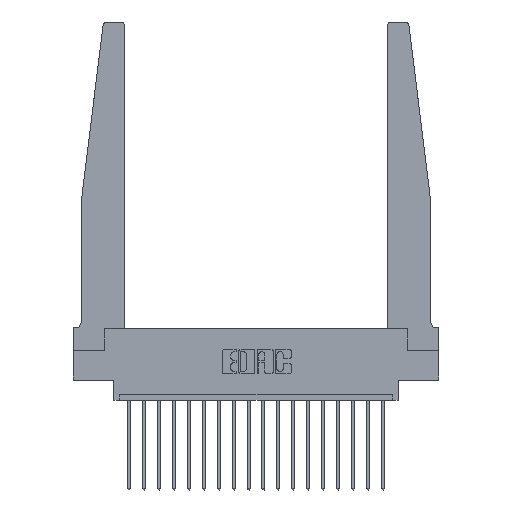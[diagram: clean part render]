
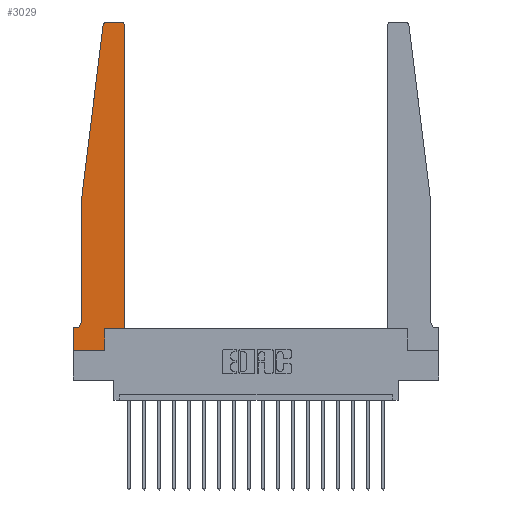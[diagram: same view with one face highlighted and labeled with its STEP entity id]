
A CAD part, top view. The second image highlights one B-rep face of the part: STEP entity #3029.
In plain terms, the highlighted planar face has unit normal (0, 0, 1).
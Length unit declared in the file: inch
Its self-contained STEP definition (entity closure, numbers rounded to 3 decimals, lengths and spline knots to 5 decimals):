
#92 = CARTESIAN_POINT ( 'NONE',  ( 0.425, 2.72, 0.37 ) ) ;
#327 = VECTOR ( 'NONE', #2339, 39.37008 ) ;
#344 = AXIS2_PLACEMENT_3D ( 'NONE', #3757, #2263, #3662 ) ;
#1224 = ORIENTED_EDGE ( 'NONE', *, *, #4427, .T. ) ;
#1246 = VECTOR ( 'NONE', #9413, 39.37008 ) ;
#1281 = CARTESIAN_POINT ( 'NONE',  ( 0.24675, 2.72367, 0.37 ) ) ;
#1677 = VERTEX_POINT ( 'NONE', #19631 ) ;
#1720 = DIRECTION ( 'NONE',  ( 1., 0., 0. ) ) ;
#2263 = DIRECTION ( 'NONE',  ( 0., 0., -1. ) ) ;
#2339 = DIRECTION ( 'NONE',  ( 1., 0., 0. ) ) ;
#2344 = EDGE_CURVE ( 'NONE', #8063, #7741, #16725, .T. ) ;
#2384 = VERTEX_POINT ( 'NONE', #13180 ) ;
#2458 = DIRECTION ( 'NONE',  ( 0., -1., 0. ) ) ;
#2871 = CARTESIAN_POINT ( 'NONE',  ( 0., 0.1875, 0.37 ) ) ;
#2964 = LINE ( 'NONE', #12581, #16701 ) ;
#2984 = CARTESIAN_POINT ( 'NONE',  ( 0.2605, 0., 0.37 ) ) ;
#3029 = ADVANCED_FACE ( 'NONE', ( #5676 ), #11694, .T. ) ;
#3662 = DIRECTION ( 'NONE',  ( -1., 0., 0. ) ) ;
#3736 = EDGE_CURVE ( 'NONE', #12469, #16454, #13163, .T. ) ;
#3757 = CARTESIAN_POINT ( 'NONE',  ( 0.015, 0.2375, 0.37 ) ) ;
#3815 = EDGE_CURVE ( 'NONE', #7389, #12259, #17255, .T. ) ;
#4425 = CARTESIAN_POINT ( 'NONE',  ( 0.065, 1.25, 0.37 ) ) ;
#4427 = EDGE_CURVE ( 'NONE', #7741, #1677, #17589, .T. ) ;
#4599 = CARTESIAN_POINT ( 'NONE',  ( 0.425, 0.18, 0.37 ) ) ;
#4727 = CARTESIAN_POINT ( 'NONE',  ( 0.065, 0.2375, 0.37 ) ) ;
#4765 = VECTOR ( 'NONE', #2458, 39.37008 ) ;
#4981 = DIRECTION ( 'NONE',  ( 1., 0., 0. ) ) ;
#5024 = ORIENTED_EDGE ( 'NONE', *, *, #12865, .T. ) ;
#5531 = CARTESIAN_POINT ( 'NONE',  ( 0., 0., 0.37 ) ) ;
#5550 = CARTESIAN_POINT ( 'NONE',  ( 0.065, 1.25, 0.37 ) ) ;
#5676 = FACE_OUTER_BOUND ( 'NONE', #5773, .T. ) ;
#5709 = VERTEX_POINT ( 'NONE', #10615 ) ;
#5773 = EDGE_LOOP ( 'NONE', ( #7231, #7520, #5024, #13146, #1224, #19653, #6195, #6059, #15503, #7593, #16820, #9755 ) ) ;
#5815 = EDGE_CURVE ( 'NONE', #7279, #14270, #15710, .T. ) ;
#6059 = ORIENTED_EDGE ( 'NONE', *, *, #3736, .T. ) ;
#6123 = LINE ( 'NONE', #4425, #13309 ) ;
#6195 = ORIENTED_EDGE ( 'NONE', *, *, #17601, .T. ) ;
#6207 = CARTESIAN_POINT ( 'NONE',  ( 0.065, 1.25, 0.37 ) ) ;
#6610 = VECTOR ( 'NONE', #15971, 39.37008 ) ;
#6934 = CARTESIAN_POINT ( 'NONE',  ( 0., 0., 0.37 ) ) ;
#7055 = CARTESIAN_POINT ( 'NONE',  ( 0.2605, 0.18, 0.37 ) ) ;
#7231 = ORIENTED_EDGE ( 'NONE', *, *, #14559, .T. ) ;
#7279 = VERTEX_POINT ( 'NONE', #92 ) ;
#7325 = EDGE_CURVE ( 'NONE', #1677, #13115, #2964, .T. ) ;
#7389 = VERTEX_POINT ( 'NONE', #7759 ) ;
#7520 = ORIENTED_EDGE ( 'NONE', *, *, #3815, .T. ) ;
#7593 = ORIENTED_EDGE ( 'NONE', *, *, #10097, .T. ) ;
#7725 = DIRECTION ( 'NONE',  ( -0.122, -0.992, 0. ) ) ;
#7741 = VERTEX_POINT ( 'NONE', #4727 ) ;
#7759 = CARTESIAN_POINT ( 'NONE',  ( 0.27653, 2.75, 0.37 ) ) ;
#8063 = VERTEX_POINT ( 'NONE', #6207 ) ;
#8451 = CARTESIAN_POINT ( 'NONE',  ( 0., 0., 0.37 ) ) ;
#8588 = DIRECTION ( 'NONE',  ( 0., 0., 1. ) ) ;
#9413 = DIRECTION ( 'NONE',  ( 0., 1., 0. ) ) ;
#9629 = DIRECTION ( 'NONE',  ( -1., 0., 0. ) ) ;
#9755 = ORIENTED_EDGE ( 'NONE', *, *, #5815, .T. ) ;
#9786 = EDGE_CURVE ( 'NONE', #16454, #2384, #14692, .T. ) ;
#10005 = VECTOR ( 'NONE', #18064, 39.37008 ) ;
#10097 = EDGE_CURVE ( 'NONE', #2384, #5709, #14643, .T. ) ;
#10288 = AXIS2_PLACEMENT_3D ( 'NONE', #12613, #19006, #4981 ) ;
#10615 = CARTESIAN_POINT ( 'NONE',  ( 0.425, 0.18, 0.37 ) ) ;
#11140 = CARTESIAN_POINT ( 'NONE',  ( 0.25, 2.75, 0.37 ) ) ;
#11694 = PLANE ( 'NONE',  #17449 ) ;
#12259 = VERTEX_POINT ( 'NONE', #1281 ) ;
#12469 = VERTEX_POINT ( 'NONE', #6934 ) ;
#12581 = CARTESIAN_POINT ( 'NONE',  ( 0.065, 0.1875, 0.37 ) ) ;
#12613 = CARTESIAN_POINT ( 'NONE',  ( 0.395, 2.72, 0.37 ) ) ;
#12865 = EDGE_CURVE ( 'NONE', #12259, #8063, #6123, .T. ) ;
#13115 = VERTEX_POINT ( 'NONE', #16531 ) ;
#13146 = ORIENTED_EDGE ( 'NONE', *, *, #2344, .T. ) ;
#13163 = LINE ( 'NONE', #5531, #327 ) ;
#13180 = CARTESIAN_POINT ( 'NONE',  ( 0.2605, 0.18, 0.37 ) ) ;
#13305 = DIRECTION ( 'NONE',  ( 1., 0., 0. ) ) ;
#13309 = VECTOR ( 'NONE', #7725, 39.37008 ) ;
#13937 = DIRECTION ( 'NONE',  ( 0., 0., 1. ) ) ;
#14270 = VERTEX_POINT ( 'NONE', #17288 ) ;
#14559 = EDGE_CURVE ( 'NONE', #14270, #7389, #18633, .T. ) ;
#14643 = LINE ( 'NONE', #19134, #17697 ) ;
#14678 = LINE ( 'NONE', #8451, #6610 ) ;
#14692 = LINE ( 'NONE', #7055, #10005 ) ;
#15503 = ORIENTED_EDGE ( 'NONE', *, *, #9786, .T. ) ;
#15710 = CIRCLE ( 'NONE', #10288, 0.03 ) ;
#15971 = DIRECTION ( 'NONE',  ( 0., -1., 0. ) ) ;
#15972 = AXIS2_PLACEMENT_3D ( 'NONE', #19636, #13937, #1720 ) ;
#16454 = VERTEX_POINT ( 'NONE', #2984 ) ;
#16531 = CARTESIAN_POINT ( 'NONE',  ( 0., 0.1875, 0.37 ) ) ;
#16701 = VECTOR ( 'NONE', #17072, 39.37008 ) ;
#16725 = LINE ( 'NONE', #5550, #4765 ) ;
#16790 = VECTOR ( 'NONE', #9629, 39.37008 ) ;
#16820 = ORIENTED_EDGE ( 'NONE', *, *, #18401, .T. ) ;
#17015 = LINE ( 'NONE', #4599, #1246 ) ;
#17072 = DIRECTION ( 'NONE',  ( -1., 0., 0. ) ) ;
#17159 = DIRECTION ( 'NONE',  ( 1., 0., 0. ) ) ;
#17255 = CIRCLE ( 'NONE', #15972, 0.03 ) ;
#17288 = CARTESIAN_POINT ( 'NONE',  ( 0.395, 2.75, 0.37 ) ) ;
#17449 = AXIS2_PLACEMENT_3D ( 'NONE', #2871, #8588, #13305 ) ;
#17589 = CIRCLE ( 'NONE', #344, 0.05 ) ;
#17601 = EDGE_CURVE ( 'NONE', #13115, #12469, #14678, .T. ) ;
#17697 = VECTOR ( 'NONE', #17159, 39.37008 ) ;
#18064 = DIRECTION ( 'NONE',  ( 0., 1., 0. ) ) ;
#18401 = EDGE_CURVE ( 'NONE', #5709, #7279, #17015, .T. ) ;
#18633 = LINE ( 'NONE', #11140, #16790 ) ;
#19006 = DIRECTION ( 'NONE',  ( 0., 0., 1. ) ) ;
#19134 = CARTESIAN_POINT ( 'NONE',  ( 0.425, 0.18, 0.37 ) ) ;
#19631 = CARTESIAN_POINT ( 'NONE',  ( 0.015, 0.1875, 0.37 ) ) ;
#19636 = CARTESIAN_POINT ( 'NONE',  ( 0.27653, 2.72, 0.37 ) ) ;
#19653 = ORIENTED_EDGE ( 'NONE', *, *, #7325, .T. ) ;
